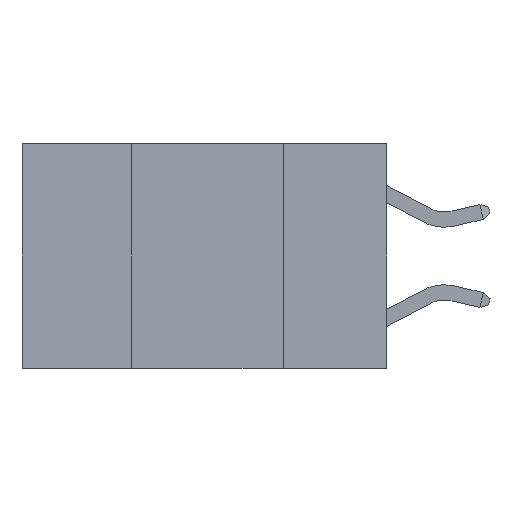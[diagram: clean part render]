
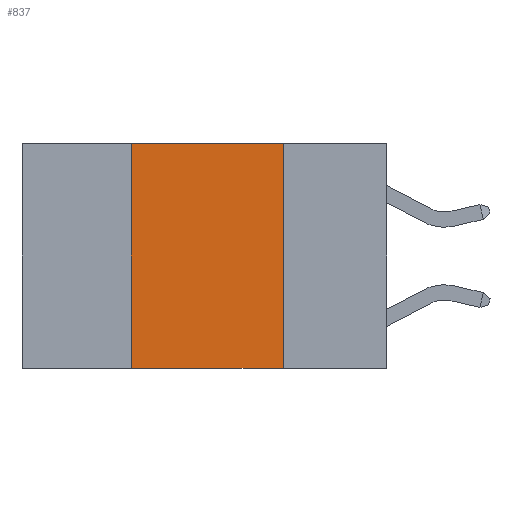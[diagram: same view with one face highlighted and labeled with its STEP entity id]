
A CAD part, left-side view. The second image highlights one B-rep face of the part: STEP entity #837.
In plain terms, the highlighted planar face has unit normal (-1, 0, 0).
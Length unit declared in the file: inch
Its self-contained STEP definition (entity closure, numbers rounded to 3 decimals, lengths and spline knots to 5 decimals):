
#497 = LINE ( 'NONE', #8836, #16181 ) ;
#597 = DIRECTION ( 'NONE',  ( 1., 0., 0. ) ) ;
#837 = ADVANCED_FACE ( 'NONE', ( #1567 ), #25042, .F. ) ;
#901 = LINE ( 'NONE', #24583, #2192 ) ;
#1567 = FACE_OUTER_BOUND ( 'NONE', #26163, .T. ) ;
#2192 = VECTOR ( 'NONE', #4240, 39.37008 ) ;
#2207 = CARTESIAN_POINT ( 'NONE',  ( 0., 0.42, 0. ) ) ;
#2917 = ORIENTED_EDGE ( 'NONE', *, *, #16319, .F. ) ;
#3996 = AXIS2_PLACEMENT_3D ( 'NONE', #12851, #597, #14913 ) ;
#4240 = DIRECTION ( 'NONE',  ( 0., -1., 0. ) ) ;
#4619 = DIRECTION ( 'NONE',  ( 0., -1., 0. ) ) ;
#5456 = VERTEX_POINT ( 'NONE', #18647 ) ;
#5914 = VERTEX_POINT ( 'NONE', #9705 ) ;
#6771 = DIRECTION ( 'NONE',  ( 0., 0., -1. ) ) ;
#7687 = ORIENTED_EDGE ( 'NONE', *, *, #12215, .F. ) ;
#8129 = LINE ( 'NONE', #24946, #23154 ) ;
#8836 = CARTESIAN_POINT ( 'NONE',  ( 0., 0.17, 0. ) ) ;
#9705 = CARTESIAN_POINT ( 'NONE',  ( 0., 0.17, -0.37 ) ) ;
#10923 = VECTOR ( 'NONE', #20569, 39.37008 ) ;
#12215 = EDGE_CURVE ( 'NONE', #5456, #5914, #497, .T. ) ;
#12804 = EDGE_CURVE ( 'NONE', #15132, #5456, #8129, .T. ) ;
#12851 = CARTESIAN_POINT ( 'NONE',  ( 0., 0.6, 0. ) ) ;
#12985 = VERTEX_POINT ( 'NONE', #17395 ) ;
#14913 = DIRECTION ( 'NONE',  ( 0., 0., -1. ) ) ;
#15132 = VERTEX_POINT ( 'NONE', #18005 ) ;
#16181 = VECTOR ( 'NONE', #6771, 39.37008 ) ;
#16319 = EDGE_CURVE ( 'NONE', #12985, #15132, #16362, .T. ) ;
#16362 = LINE ( 'NONE', #2207, #10923 ) ;
#17395 = CARTESIAN_POINT ( 'NONE',  ( 0., 0.42, -0.37 ) ) ;
#18005 = CARTESIAN_POINT ( 'NONE',  ( 0., 0.42, 0. ) ) ;
#18355 = EDGE_CURVE ( 'NONE', #12985, #5914, #901, .T. ) ;
#18562 = ORIENTED_EDGE ( 'NONE', *, *, #12804, .F. ) ;
#18647 = CARTESIAN_POINT ( 'NONE',  ( 0., 0.17, 0. ) ) ;
#19199 = ORIENTED_EDGE ( 'NONE', *, *, #18355, .T. ) ;
#20569 = DIRECTION ( 'NONE',  ( 0., 0., 1. ) ) ;
#23154 = VECTOR ( 'NONE', #4619, 39.37008 ) ;
#24583 = CARTESIAN_POINT ( 'NONE',  ( 0., 0.6, -0.37 ) ) ;
#24946 = CARTESIAN_POINT ( 'NONE',  ( 0., 0.6, 0. ) ) ;
#25042 = PLANE ( 'NONE',  #3996 ) ;
#26163 = EDGE_LOOP ( 'NONE', ( #7687, #18562, #2917, #19199 ) ) ;
